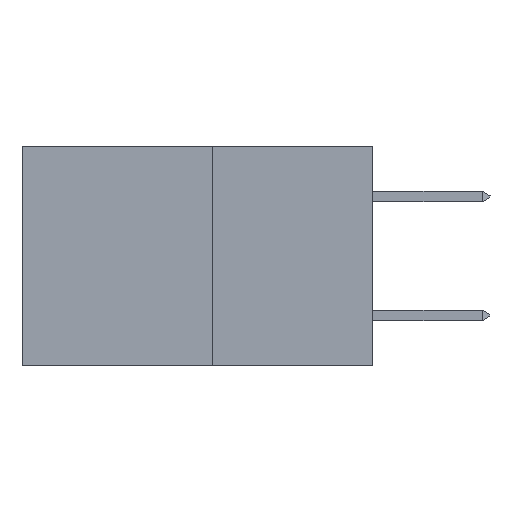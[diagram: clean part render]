
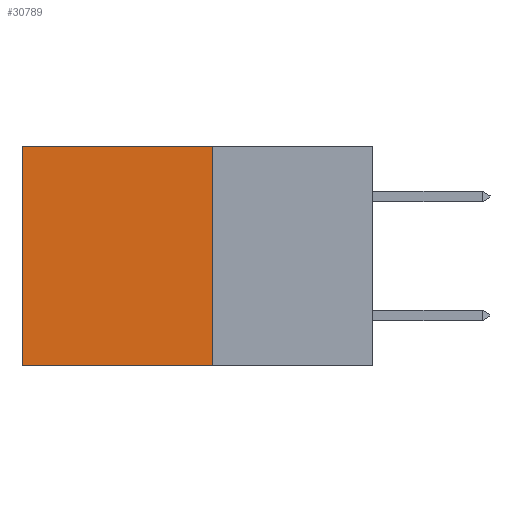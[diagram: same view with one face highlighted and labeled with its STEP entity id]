
A CAD part, left-side view. The second image highlights one B-rep face of the part: STEP entity #30789.
In plain terms, the highlighted planar face has unit normal (-1, 0, 0).
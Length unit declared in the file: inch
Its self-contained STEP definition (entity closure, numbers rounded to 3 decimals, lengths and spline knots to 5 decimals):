
#154 = EDGE_CURVE ( 'NONE', #24224, #8382, #13481, .T. ) ;
#412 = EDGE_CURVE ( 'NONE', #8382, #24519, #12206, .T. ) ;
#715 = CARTESIAN_POINT ( 'NONE',  ( 0.277, 0.27, -0.37 ) ) ;
#1703 = AXIS2_PLACEMENT_3D ( 'NONE', #715, #3415, #22169 ) ;
#1980 = ORIENTED_EDGE ( 'NONE', *, *, #10607, .F. ) ;
#2960 = ORIENTED_EDGE ( 'NONE', *, *, #16317, .F. ) ;
#3113 = VERTEX_POINT ( 'NONE', #23611 ) ;
#3415 = DIRECTION ( 'NONE',  ( 1., 0., 0. ) ) ;
#3626 = CARTESIAN_POINT ( 'NONE',  ( 0.277, 0.59, 0. ) ) ;
#4231 = VECTOR ( 'NONE', #17668, 39.37008 ) ;
#7674 = LINE ( 'NONE', #28568, #28923 ) ;
#8101 = CARTESIAN_POINT ( 'NONE',  ( 0.277, 0.27, 0. ) ) ;
#8382 = VERTEX_POINT ( 'NONE', #3626 ) ;
#9697 = CARTESIAN_POINT ( 'NONE',  ( 0.277, 0.27, -0.37 ) ) ;
#10607 = EDGE_CURVE ( 'NONE', #3113, #24519, #7674, .T. ) ;
#12206 = LINE ( 'NONE', #17933, #4231 ) ;
#13463 = CARTESIAN_POINT ( 'NONE',  ( 0.277, 0.27, 0. ) ) ;
#13481 = LINE ( 'NONE', #13463, #18905 ) ;
#13838 = DIRECTION ( 'NONE',  ( 0., 1., 0. ) ) ;
#16317 = EDGE_CURVE ( 'NONE', #24224, #3113, #26918, .T. ) ;
#16794 = PLANE ( 'NONE',  #1703 ) ;
#17668 = DIRECTION ( 'NONE',  ( 0., 0., -1. ) ) ;
#17933 = CARTESIAN_POINT ( 'NONE',  ( 0.277, 0.59, -0.37 ) ) ;
#18021 = ORIENTED_EDGE ( 'NONE', *, *, #154, .T. ) ;
#18905 = VECTOR ( 'NONE', #13838, 39.37008 ) ;
#19602 = CARTESIAN_POINT ( 'NONE',  ( 0.277, 0.59, -0.37 ) ) ;
#22169 = DIRECTION ( 'NONE',  ( 0., 0., -1. ) ) ;
#23611 = CARTESIAN_POINT ( 'NONE',  ( 0.277, 0.27, -0.37 ) ) ;
#24224 = VERTEX_POINT ( 'NONE', #8101 ) ;
#24519 = VERTEX_POINT ( 'NONE', #19602 ) ;
#26918 = LINE ( 'NONE', #9697, #33034 ) ;
#28568 = CARTESIAN_POINT ( 'NONE',  ( 0.277, 0.27, -0.37 ) ) ;
#28923 = VECTOR ( 'NONE', #31171, 39.37008 ) ;
#30789 = ADVANCED_FACE ( 'NONE', ( #34215 ), #16794, .F. ) ;
#30922 = DIRECTION ( 'NONE',  ( 0., 0., -1. ) ) ;
#31171 = DIRECTION ( 'NONE',  ( 0., 1., 0. ) ) ;
#32911 = EDGE_LOOP ( 'NONE', ( #33499, #1980, #2960, #18021 ) ) ;
#33034 = VECTOR ( 'NONE', #30922, 39.37008 ) ;
#33499 = ORIENTED_EDGE ( 'NONE', *, *, #412, .T. ) ;
#34215 = FACE_OUTER_BOUND ( 'NONE', #32911, .T. ) ;
